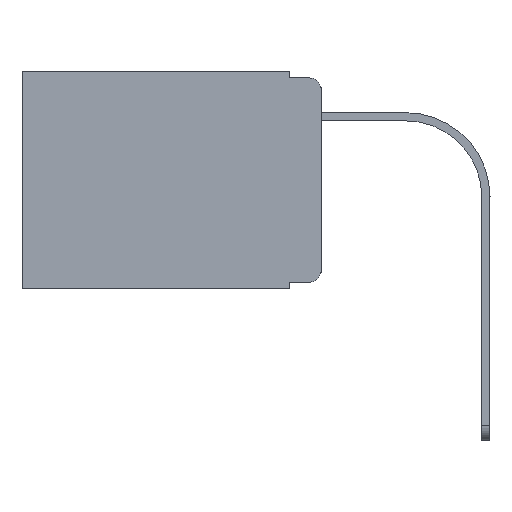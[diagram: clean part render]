
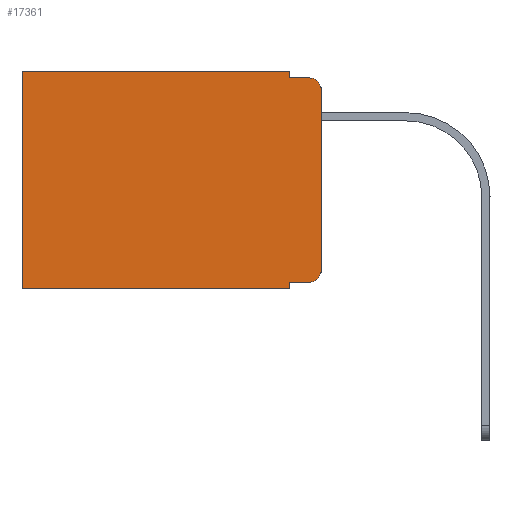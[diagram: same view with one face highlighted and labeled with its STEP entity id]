
A CAD part, left-side view. The second image highlights one B-rep face of the part: STEP entity #17361.
In plain terms, the highlighted planar face has unit normal (-1, 0, 0).
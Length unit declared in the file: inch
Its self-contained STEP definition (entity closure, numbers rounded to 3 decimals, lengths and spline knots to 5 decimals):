
#113 = EDGE_CURVE ( 'NONE', #10380, #22488, #5009, .T. ) ;
#819 = EDGE_CURVE ( 'NONE', #12976, #21744, #1177, .T. ) ;
#873 = EDGE_LOOP ( 'NONE', ( #16084, #12505, #17380, #12914, #9423, #3266, #5977, #13296, #6583, #12859 ) ) ;
#1177 = LINE ( 'NONE', #11597, #8304 ) ;
#1475 = DIRECTION ( 'NONE',  ( 0., 0., -1. ) ) ;
#1786 = CARTESIAN_POINT ( 'NONE',  ( 0.298, 0.02, -0.01 ) ) ;
#1825 = DIRECTION ( 'NONE',  ( 0., -1., 0. ) ) ;
#1853 = DIRECTION ( 'NONE',  ( 0., 0., -1. ) ) ;
#1860 = CARTESIAN_POINT ( 'NONE',  ( 0.298, 0.02, -0.313 ) ) ;
#2084 = PLANE ( 'NONE',  #9948 ) ;
#2256 = VECTOR ( 'NONE', #1475, 39.37008 ) ;
#2574 = EDGE_CURVE ( 'NONE', #21744, #15131, #9467, .T. ) ;
#3266 = ORIENTED_EDGE ( 'NONE', *, *, #2574, .T. ) ;
#4747 = EDGE_CURVE ( 'NONE', #9239, #8885, #17799, .T. ) ;
#5009 = LINE ( 'NONE', #5340, #9210 ) ;
#5280 = EDGE_CURVE ( 'NONE', #10380, #10582, #14375, .T. ) ;
#5340 = CARTESIAN_POINT ( 'NONE',  ( 0.298, 0.051, 0. ) ) ;
#5381 = VECTOR ( 'NONE', #12960, 39.37008 ) ;
#5393 = CARTESIAN_POINT ( 'NONE',  ( 0.298, 0.02, -0.03 ) ) ;
#5619 = DIRECTION ( 'NONE',  ( -1., 0., 0. ) ) ;
#5872 = EDGE_CURVE ( 'NONE', #9239, #23254, #13543, .T. ) ;
#5977 = ORIENTED_EDGE ( 'NONE', *, *, #6730, .F. ) ;
#6583 = ORIENTED_EDGE ( 'NONE', *, *, #5280, .T. ) ;
#6730 = EDGE_CURVE ( 'NONE', #22488, #15131, #18782, .T. ) ;
#7172 = DIRECTION ( 'NONE',  ( 1., 0., 0. ) ) ;
#7523 = FACE_OUTER_BOUND ( 'NONE', #873, .T. ) ;
#7577 = AXIS2_PLACEMENT_3D ( 'NONE', #5393, #5619, #1853 ) ;
#7631 = LINE ( 'NONE', #21838, #5381 ) ;
#7734 = VECTOR ( 'NONE', #15212, 39.37008 ) ;
#7985 = CARTESIAN_POINT ( 'NONE',  ( 0.298, 0.051, -0.01 ) ) ;
#8146 = EDGE_CURVE ( 'NONE', #10582, #23254, #12212, .T. ) ;
#8304 = VECTOR ( 'NONE', #15389, 39.37008 ) ;
#8587 = CARTESIAN_POINT ( 'NONE',  ( 0.298, 0.051, -0.01 ) ) ;
#8817 = CARTESIAN_POINT ( 'NONE',  ( 0.298, 0.051, -0.333 ) ) ;
#8819 = CARTESIAN_POINT ( 'NONE',  ( 0.298, 0.473, 0. ) ) ;
#8885 = VERTEX_POINT ( 'NONE', #1786 ) ;
#9210 = VECTOR ( 'NONE', #19473, 39.37008 ) ;
#9239 = VERTEX_POINT ( 'NONE', #13968 ) ;
#9423 = ORIENTED_EDGE ( 'NONE', *, *, #819, .T. ) ;
#9467 = LINE ( 'NONE', #8819, #2256 ) ;
#9752 = CARTESIAN_POINT ( 'NONE',  ( 0.298, 0., 0. ) ) ;
#9820 = CARTESIAN_POINT ( 'NONE',  ( 0.298, 0., -0.313 ) ) ;
#9948 = AXIS2_PLACEMENT_3D ( 'NONE', #12844, #7172, #20068 ) ;
#10108 = EDGE_CURVE ( 'NONE', #22480, #8885, #22418, .T. ) ;
#10321 = CARTESIAN_POINT ( 'NONE',  ( 0.298, 0.473, -0.343 ) ) ;
#10380 = VERTEX_POINT ( 'NONE', #8817 ) ;
#10506 = CARTESIAN_POINT ( 'NONE',  ( 0.298, 0.051, 0. ) ) ;
#10582 = VERTEX_POINT ( 'NONE', #22158 ) ;
#11597 = CARTESIAN_POINT ( 'NONE',  ( 0.298, 0., 0. ) ) ;
#12212 = CIRCLE ( 'NONE', #14105, 0.02 ) ;
#12505 = ORIENTED_EDGE ( 'NONE', *, *, #4747, .T. ) ;
#12844 = CARTESIAN_POINT ( 'NONE',  ( 0.298, 0., 0. ) ) ;
#12859 = ORIENTED_EDGE ( 'NONE', *, *, #8146, .T. ) ;
#12914 = ORIENTED_EDGE ( 'NONE', *, *, #17360, .F. ) ;
#12960 = DIRECTION ( 'NONE',  ( 0., 0., -1. ) ) ;
#12976 = VERTEX_POINT ( 'NONE', #10506 ) ;
#13296 = ORIENTED_EDGE ( 'NONE', *, *, #113, .F. ) ;
#13543 = LINE ( 'NONE', #9752, #14072 ) ;
#13968 = CARTESIAN_POINT ( 'NONE',  ( 0.298, 0., -0.03 ) ) ;
#14072 = VECTOR ( 'NONE', #16963, 39.37008 ) ;
#14105 = AXIS2_PLACEMENT_3D ( 'NONE', #1860, #21857, #16087 ) ;
#14375 = LINE ( 'NONE', #19834, #15932 ) ;
#15131 = VERTEX_POINT ( 'NONE', #10321 ) ;
#15212 = DIRECTION ( 'NONE',  ( 0., -1., 0. ) ) ;
#15389 = DIRECTION ( 'NONE',  ( 0., 1., 0. ) ) ;
#15796 = CARTESIAN_POINT ( 'NONE',  ( 0.298, 0.051, -0.343 ) ) ;
#15932 = VECTOR ( 'NONE', #1825, 39.37008 ) ;
#16084 = ORIENTED_EDGE ( 'NONE', *, *, #5872, .F. ) ;
#16087 = DIRECTION ( 'NONE',  ( 0., 0., -1. ) ) ;
#16963 = DIRECTION ( 'NONE',  ( 0., 0., -1. ) ) ;
#17139 = CARTESIAN_POINT ( 'NONE',  ( 0.298, 0.473, 0. ) ) ;
#17360 = EDGE_CURVE ( 'NONE', #12976, #22480, #7631, .T. ) ;
#17361 = ADVANCED_FACE ( 'NONE', ( #7523 ), #2084, .F. ) ;
#17380 = ORIENTED_EDGE ( 'NONE', *, *, #10108, .F. ) ;
#17799 = CIRCLE ( 'NONE', #7577, 0.02 ) ;
#18243 = VECTOR ( 'NONE', #18889, 39.37008 ) ;
#18782 = LINE ( 'NONE', #19144, #18243 ) ;
#18889 = DIRECTION ( 'NONE',  ( 0., 1., 0. ) ) ;
#19144 = CARTESIAN_POINT ( 'NONE',  ( 0.298, 0., -0.343 ) ) ;
#19473 = DIRECTION ( 'NONE',  ( 0., 0., -1. ) ) ;
#19834 = CARTESIAN_POINT ( 'NONE',  ( 0.298, 0.051, -0.333 ) ) ;
#20068 = DIRECTION ( 'NONE',  ( 0., 0., -1. ) ) ;
#21744 = VERTEX_POINT ( 'NONE', #17139 ) ;
#21838 = CARTESIAN_POINT ( 'NONE',  ( 0.298, 0.051, 0. ) ) ;
#21857 = DIRECTION ( 'NONE',  ( -1., 0., 0. ) ) ;
#22158 = CARTESIAN_POINT ( 'NONE',  ( 0.298, 0.02, -0.333 ) ) ;
#22418 = LINE ( 'NONE', #7985, #7734 ) ;
#22480 = VERTEX_POINT ( 'NONE', #8587 ) ;
#22488 = VERTEX_POINT ( 'NONE', #15796 ) ;
#23254 = VERTEX_POINT ( 'NONE', #9820 ) ;
